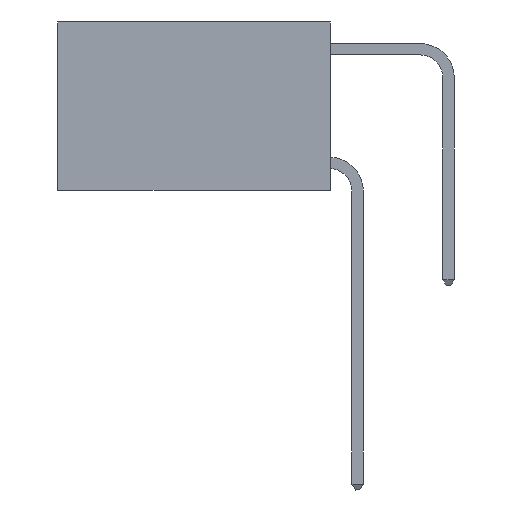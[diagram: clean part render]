
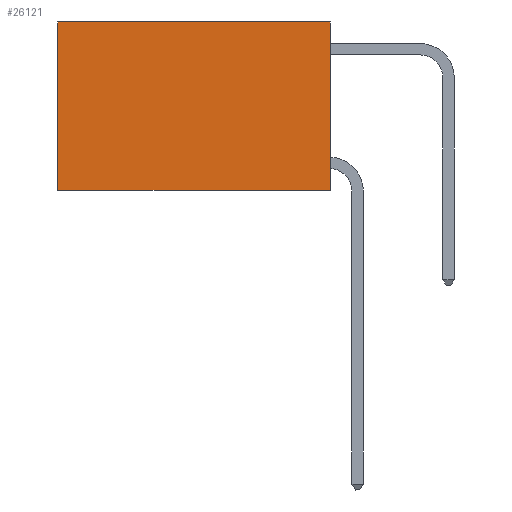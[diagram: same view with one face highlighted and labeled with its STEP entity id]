
A CAD part, left-side view. The second image highlights one B-rep face of the part: STEP entity #26121.
In plain terms, the highlighted planar face has unit normal (-1, 0, 0).
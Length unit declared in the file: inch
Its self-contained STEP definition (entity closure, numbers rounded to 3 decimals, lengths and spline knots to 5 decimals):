
#2377 = VECTOR ( 'NONE', #15985, 39.37008 ) ;
#2457 = VECTOR ( 'NONE', #12978, 39.37008 ) ;
#3046 = EDGE_CURVE ( 'NONE', #22851, #19977, #26523, .T. ) ;
#3108 = ORIENTED_EDGE ( 'NONE', *, *, #3046, .T. ) ;
#3874 = LINE ( 'NONE', #23323, #15628 ) ;
#4285 = FACE_OUTER_BOUND ( 'NONE', #15546, .T. ) ;
#5045 = VERTEX_POINT ( 'NONE', #23783 ) ;
#8266 = LINE ( 'NONE', #13794, #2377 ) ;
#8767 = AXIS2_PLACEMENT_3D ( 'NONE', #15266, #26241, #13140 ) ;
#9276 = CARTESIAN_POINT ( 'NONE',  ( 0.2625, 0., 0. ) ) ;
#10225 = VECTOR ( 'NONE', #11879, 39.37008 ) ;
#10905 = ORIENTED_EDGE ( 'NONE', *, *, #27293, .T. ) ;
#11786 = CARTESIAN_POINT ( 'NONE',  ( 0.2625, 0., 0. ) ) ;
#11879 = DIRECTION ( 'NONE',  ( 0., 0., -1. ) ) ;
#12978 = DIRECTION ( 'NONE',  ( 0., 0., -1. ) ) ;
#13052 = VERTEX_POINT ( 'NONE', #9276 ) ;
#13140 = DIRECTION ( 'NONE',  ( 0., 0., -1. ) ) ;
#13441 = ORIENTED_EDGE ( 'NONE', *, *, #16122, .F. ) ;
#13794 = CARTESIAN_POINT ( 'NONE',  ( 0.2625, 0., -0.37 ) ) ;
#14635 = DIRECTION ( 'NONE',  ( 0., 1., 0. ) ) ;
#15266 = CARTESIAN_POINT ( 'NONE',  ( 0.2625, 0., 0. ) ) ;
#15546 = EDGE_LOOP ( 'NONE', ( #3108, #13441, #27783, #10905 ) ) ;
#15628 = VECTOR ( 'NONE', #14635, 39.37008 ) ;
#15985 = DIRECTION ( 'NONE',  ( 0., 1., 0. ) ) ;
#16084 = LINE ( 'NONE', #11786, #10225 ) ;
#16122 = EDGE_CURVE ( 'NONE', #5045, #19977, #8266, .T. ) ;
#17587 = EDGE_CURVE ( 'NONE', #13052, #5045, #16084, .T. ) ;
#19569 = CARTESIAN_POINT ( 'NONE',  ( 0.2625, 0.6, 0. ) ) ;
#19977 = VERTEX_POINT ( 'NONE', #22044 ) ;
#22044 = CARTESIAN_POINT ( 'NONE',  ( 0.2625, 0.6, -0.37 ) ) ;
#22851 = VERTEX_POINT ( 'NONE', #25137 ) ;
#23323 = CARTESIAN_POINT ( 'NONE',  ( 0.2625, 0., 0. ) ) ;
#23783 = CARTESIAN_POINT ( 'NONE',  ( 0.2625, 0., -0.37 ) ) ;
#24049 = PLANE ( 'NONE',  #8767 ) ;
#25137 = CARTESIAN_POINT ( 'NONE',  ( 0.2625, 0.6, 0. ) ) ;
#26121 = ADVANCED_FACE ( 'NONE', ( #4285 ), #24049, .F. ) ;
#26241 = DIRECTION ( 'NONE',  ( 1., 0., 0. ) ) ;
#26523 = LINE ( 'NONE', #19569, #2457 ) ;
#27293 = EDGE_CURVE ( 'NONE', #13052, #22851, #3874, .T. ) ;
#27783 = ORIENTED_EDGE ( 'NONE', *, *, #17587, .F. ) ;
